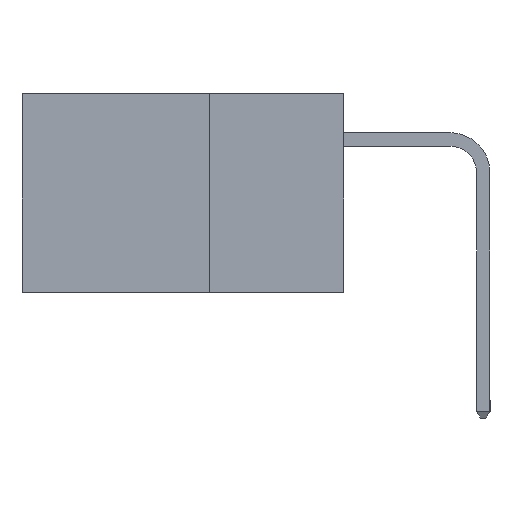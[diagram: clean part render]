
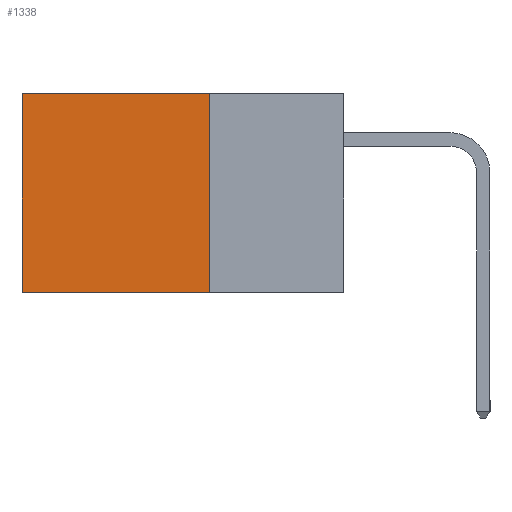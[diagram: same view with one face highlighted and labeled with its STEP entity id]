
A CAD part, left-side view. The second image highlights one B-rep face of the part: STEP entity #1338.
In plain terms, the highlighted planar face has unit normal (-1, 0, 0).
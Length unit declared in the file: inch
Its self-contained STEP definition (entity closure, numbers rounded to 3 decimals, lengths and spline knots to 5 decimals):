
#84 = VECTOR ( 'NONE', #3178, 39.37008 ) ;
#1338 = ADVANCED_FACE ( 'NONE', ( #2207 ), #7449, .F. ) ;
#1751 = VERTEX_POINT ( 'NONE', #3465 ) ;
#2011 = EDGE_CURVE ( 'NONE', #1751, #2918, #9683, .T. ) ;
#2207 = FACE_OUTER_BOUND ( 'NONE', #11229, .T. ) ;
#2346 = CARTESIAN_POINT ( 'NONE',  ( 0.2615, 0.25, 0. ) ) ;
#2673 = VECTOR ( 'NONE', #7576, 39.37008 ) ;
#2805 = AXIS2_PLACEMENT_3D ( 'NONE', #7616, #7422, #7394 ) ;
#2854 = LINE ( 'NONE', #5069, #84 ) ;
#2918 = VERTEX_POINT ( 'NONE', #9439 ) ;
#3178 = DIRECTION ( 'NONE',  ( 0., 0., -1. ) ) ;
#3201 = LINE ( 'NONE', #7521, #5429 ) ;
#3465 = CARTESIAN_POINT ( 'NONE',  ( 0.2615, 0.25, -0.37 ) ) ;
#3471 = CARTESIAN_POINT ( 'NONE',  ( 0.2615, 0.25, 0. ) ) ;
#4427 = DIRECTION ( 'NONE',  ( 0., 1., 0. ) ) ;
#5069 = CARTESIAN_POINT ( 'NONE',  ( 0.2615, 0.25, -0.37 ) ) ;
#5429 = VECTOR ( 'NONE', #11868, 39.37008 ) ;
#5832 = ORIENTED_EDGE ( 'NONE', *, *, #10622, .T. ) ;
#5849 = ORIENTED_EDGE ( 'NONE', *, *, #7021, .T. ) ;
#5985 = ORIENTED_EDGE ( 'NONE', *, *, #2011, .F. ) ;
#5999 = VECTOR ( 'NONE', #4427, 39.37008 ) ;
#6046 = ORIENTED_EDGE ( 'NONE', *, *, #11043, .F. ) ;
#6230 = VERTEX_POINT ( 'NONE', #11683 ) ;
#6697 = VERTEX_POINT ( 'NONE', #2346 ) ;
#7021 = EDGE_CURVE ( 'NONE', #6230, #2918, #3201, .T. ) ;
#7394 = DIRECTION ( 'NONE',  ( 0., 0., -1. ) ) ;
#7422 = DIRECTION ( 'NONE',  ( 1., 0., 0. ) ) ;
#7449 = PLANE ( 'NONE',  #2805 ) ;
#7521 = CARTESIAN_POINT ( 'NONE',  ( 0.2615, 0.6, -0.37 ) ) ;
#7576 = DIRECTION ( 'NONE',  ( 0., 1., 0. ) ) ;
#7616 = CARTESIAN_POINT ( 'NONE',  ( 0.2615, 0.25, -0.37 ) ) ;
#8309 = LINE ( 'NONE', #3471, #5999 ) ;
#9439 = CARTESIAN_POINT ( 'NONE',  ( 0.2615, 0.6, -0.37 ) ) ;
#9683 = LINE ( 'NONE', #11297, #2673 ) ;
#10622 = EDGE_CURVE ( 'NONE', #6697, #6230, #8309, .T. ) ;
#11043 = EDGE_CURVE ( 'NONE', #6697, #1751, #2854, .T. ) ;
#11229 = EDGE_LOOP ( 'NONE', ( #5849, #5985, #6046, #5832 ) ) ;
#11297 = CARTESIAN_POINT ( 'NONE',  ( 0.2615, 0.25, -0.37 ) ) ;
#11683 = CARTESIAN_POINT ( 'NONE',  ( 0.2615, 0.6, 0. ) ) ;
#11868 = DIRECTION ( 'NONE',  ( 0., 0., -1. ) ) ;
